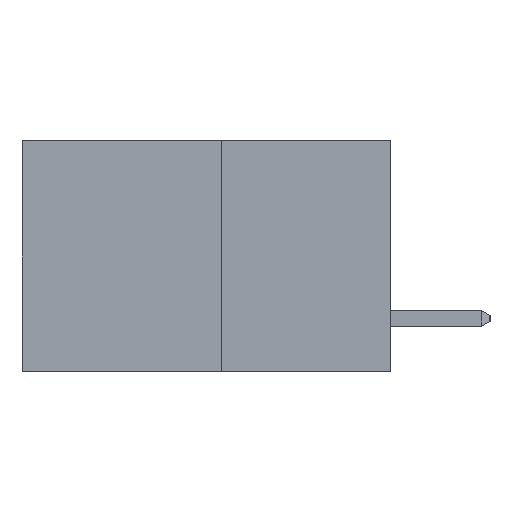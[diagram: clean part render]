
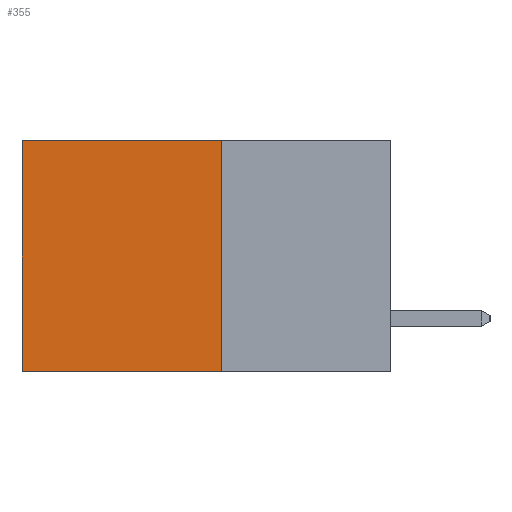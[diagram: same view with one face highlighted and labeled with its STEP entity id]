
A CAD part, left-side view. The second image highlights one B-rep face of the part: STEP entity #355.
In plain terms, the highlighted planar face has unit normal (-1, 0, 0).
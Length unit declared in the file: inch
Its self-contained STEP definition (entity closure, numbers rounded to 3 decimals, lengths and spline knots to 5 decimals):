
#14 = CARTESIAN_POINT ( 'NONE',  ( 0.277, 0.27, 0. ) ) ;
#133 = LINE ( 'NONE', #12347, #8312 ) ;
#355 = ADVANCED_FACE ( 'NONE', ( #8449 ), #3261, .F. ) ;
#593 = AXIS2_PLACEMENT_3D ( 'NONE', #1877, #14116, #18884 ) ;
#704 = EDGE_CURVE ( 'NONE', #13266, #5129, #18532, .T. ) ;
#1877 = CARTESIAN_POINT ( 'NONE',  ( 0.277, 0.27, -0.37 ) ) ;
#3256 = CARTESIAN_POINT ( 'NONE',  ( 0.277, 0.59, 0. ) ) ;
#3261 = PLANE ( 'NONE',  #593 ) ;
#4483 = VECTOR ( 'NONE', #13855, 39.37008 ) ;
#5129 = VERTEX_POINT ( 'NONE', #13113 ) ;
#5740 = VECTOR ( 'NONE', #10166, 39.37008 ) ;
#6088 = EDGE_CURVE ( 'NONE', #11008, #5129, #8715, .T. ) ;
#6169 = CARTESIAN_POINT ( 'NONE',  ( 0.277, 0.59, -0.37 ) ) ;
#6192 = DIRECTION ( 'NONE',  ( 0., 0., -1. ) ) ;
#8312 = VECTOR ( 'NONE', #13980, 39.37008 ) ;
#8449 = FACE_OUTER_BOUND ( 'NONE', #9872, .T. ) ;
#8523 = CARTESIAN_POINT ( 'NONE',  ( 0.277, 0.27, 0. ) ) ;
#8715 = LINE ( 'NONE', #18588, #4483 ) ;
#9872 = EDGE_LOOP ( 'NONE', ( #20447, #11944, #18644, #18268 ) ) ;
#10141 = EDGE_CURVE ( 'NONE', #20766, #11008, #133, .T. ) ;
#10166 = DIRECTION ( 'NONE',  ( 0., 1., 0. ) ) ;
#11008 = VERTEX_POINT ( 'NONE', #11423 ) ;
#11423 = CARTESIAN_POINT ( 'NONE',  ( 0.277, 0.27, -0.37 ) ) ;
#11944 = ORIENTED_EDGE ( 'NONE', *, *, #6088, .F. ) ;
#12347 = CARTESIAN_POINT ( 'NONE',  ( 0.277, 0.27, -0.37 ) ) ;
#13113 = CARTESIAN_POINT ( 'NONE',  ( 0.277, 0.59, -0.37 ) ) ;
#13266 = VERTEX_POINT ( 'NONE', #3256 ) ;
#13855 = DIRECTION ( 'NONE',  ( 0., 1., 0. ) ) ;
#13980 = DIRECTION ( 'NONE',  ( 0., 0., -1. ) ) ;
#14116 = DIRECTION ( 'NONE',  ( 1., 0., 0. ) ) ;
#15197 = EDGE_CURVE ( 'NONE', #20766, #13266, #18598, .T. ) ;
#18033 = VECTOR ( 'NONE', #6192, 39.37008 ) ;
#18268 = ORIENTED_EDGE ( 'NONE', *, *, #15197, .T. ) ;
#18532 = LINE ( 'NONE', #6169, #18033 ) ;
#18588 = CARTESIAN_POINT ( 'NONE',  ( 0.277, 0.27, -0.37 ) ) ;
#18598 = LINE ( 'NONE', #8523, #5740 ) ;
#18644 = ORIENTED_EDGE ( 'NONE', *, *, #10141, .F. ) ;
#18884 = DIRECTION ( 'NONE',  ( 0., 0., -1. ) ) ;
#20447 = ORIENTED_EDGE ( 'NONE', *, *, #704, .T. ) ;
#20766 = VERTEX_POINT ( 'NONE', #14 ) ;
